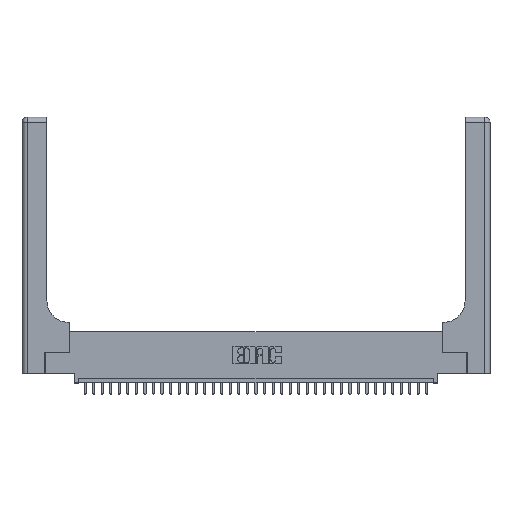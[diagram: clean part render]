
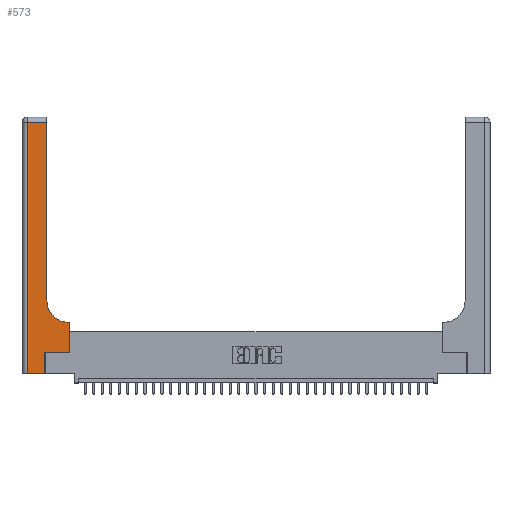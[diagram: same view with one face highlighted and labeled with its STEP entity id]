
A CAD part, top view. The second image highlights one B-rep face of the part: STEP entity #573.
In plain terms, the highlighted planar face has unit normal (0, 0, 1).
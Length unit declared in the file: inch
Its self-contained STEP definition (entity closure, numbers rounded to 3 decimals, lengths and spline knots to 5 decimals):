
#573 = ADVANCED_FACE ( 'NONE', ( #34009 ), #28757, .F. ) ;
#732 = DIRECTION ( 'NONE',  ( 0., 1., 0. ) ) ;
#1636 = VECTOR ( 'NONE', #17524, 39.37008 ) ;
#2463 = CARTESIAN_POINT ( 'NONE',  ( 0.06, 2.94, 0.37 ) ) ;
#3347 = DIRECTION ( 'NONE',  ( 0., -1., 0. ) ) ;
#3861 = CARTESIAN_POINT ( 'NONE',  ( 0.269, 0., 0.37 ) ) ;
#3871 = DIRECTION ( 'NONE',  ( 0., 0., -1. ) ) ;
#4919 = DIRECTION ( 'NONE',  ( 0., 0., -1. ) ) ;
#5036 = CARTESIAN_POINT ( 'NONE',  ( 0.5415, 0.6, 0.37 ) ) ;
#5107 = ORIENTED_EDGE ( 'NONE', *, *, #7528, .T. ) ;
#5230 = EDGE_CURVE ( 'NONE', #20240, #35021, #26653, .T. ) ;
#5284 = CARTESIAN_POINT ( 'NONE',  ( 0.5415, 0.85, 0.37 ) ) ;
#5801 = CARTESIAN_POINT ( 'NONE',  ( 0.269, 0.25, 0.37 ) ) ;
#6693 = CARTESIAN_POINT ( 'NONE',  ( 0.5585, 0.25, 0.37 ) ) ;
#7074 = EDGE_CURVE ( 'NONE', #24769, #20240, #18142, .T. ) ;
#7220 = CARTESIAN_POINT ( 'NONE',  ( 0.2915, 0.85, 0.37 ) ) ;
#7409 = EDGE_LOOP ( 'NONE', ( #34728, #28143, #26007, #19621, #34927, #36185, #23797, #20882, #5107 ) ) ;
#7528 = EDGE_CURVE ( 'NONE', #23286, #25486, #25134, .T. ) ;
#8420 = LINE ( 'NONE', #15697, #35168 ) ;
#8437 = CARTESIAN_POINT ( 'NONE',  ( 0., 0., 0.37 ) ) ;
#8805 = DIRECTION ( 'NONE',  ( -1., 0., 0. ) ) ;
#10621 = DIRECTION ( 'NONE',  ( 1., 0., 0. ) ) ;
#10842 = EDGE_CURVE ( 'NONE', #25486, #23081, #34946, .T. ) ;
#12001 = DIRECTION ( 'NONE',  ( 0., 1., 0. ) ) ;
#14422 = VECTOR ( 'NONE', #12001, 39.37008 ) ;
#14959 = DIRECTION ( 'NONE',  ( -1., 0., 0. ) ) ;
#15079 = CARTESIAN_POINT ( 'NONE',  ( 0., 3., 0.37 ) ) ;
#15422 = EDGE_CURVE ( 'NONE', #32567, #24769, #21526, .T. ) ;
#15676 = DIRECTION ( 'NONE',  ( 1., 0., 0. ) ) ;
#15697 = CARTESIAN_POINT ( 'NONE',  ( 0., 2.94, 0.37 ) ) ;
#16866 = EDGE_CURVE ( 'NONE', #35021, #20359, #33232, .T. ) ;
#17463 = LINE ( 'NONE', #6693, #18391 ) ;
#17524 = DIRECTION ( 'NONE',  ( 1., 0., 0. ) ) ;
#17814 = CARTESIAN_POINT ( 'NONE',  ( 0.2915, 3., 0.37 ) ) ;
#18142 = LINE ( 'NONE', #8437, #30452 ) ;
#18391 = VECTOR ( 'NONE', #26775, 39.37008 ) ;
#19621 = ORIENTED_EDGE ( 'NONE', *, *, #7074, .T. ) ;
#20240 = VERTEX_POINT ( 'NONE', #3861 ) ;
#20359 = VERTEX_POINT ( 'NONE', #24331 ) ;
#20882 = ORIENTED_EDGE ( 'NONE', *, *, #34352, .T. ) ;
#21526 = LINE ( 'NONE', #35166, #31147 ) ;
#21652 = EDGE_CURVE ( 'NONE', #23081, #32567, #8420, .T. ) ;
#22621 = CARTESIAN_POINT ( 'NONE',  ( 0.5585, 0.6, 0.37 ) ) ;
#23081 = VERTEX_POINT ( 'NONE', #34076 ) ;
#23286 = VERTEX_POINT ( 'NONE', #5036 ) ;
#23545 = CARTESIAN_POINT ( 'NONE',  ( 0.269, 0., 0.37 ) ) ;
#23676 = EDGE_CURVE ( 'NONE', #20359, #28381, #17463, .T. ) ;
#23797 = ORIENTED_EDGE ( 'NONE', *, *, #23676, .T. ) ;
#24331 = CARTESIAN_POINT ( 'NONE',  ( 0.5585, 0.25, 0.37 ) ) ;
#24769 = VERTEX_POINT ( 'NONE', #27180 ) ;
#25134 = CIRCLE ( 'NONE', #28511, 0.25 ) ;
#25486 = VERTEX_POINT ( 'NONE', #7220 ) ;
#26007 = ORIENTED_EDGE ( 'NONE', *, *, #15422, .T. ) ;
#26653 = LINE ( 'NONE', #23545, #29741 ) ;
#26775 = DIRECTION ( 'NONE',  ( 0., 1., 0. ) ) ;
#27180 = CARTESIAN_POINT ( 'NONE',  ( 0.06, 0., 0.37 ) ) ;
#28143 = ORIENTED_EDGE ( 'NONE', *, *, #21652, .T. ) ;
#28381 = VERTEX_POINT ( 'NONE', #22621 ) ;
#28511 = AXIS2_PLACEMENT_3D ( 'NONE', #5284, #4919, #10621 ) ;
#28757 = PLANE ( 'NONE',  #32927 ) ;
#29741 = VECTOR ( 'NONE', #732, 39.37008 ) ;
#29873 = DIRECTION ( 'NONE',  ( -1., 0., 0. ) ) ;
#30452 = VECTOR ( 'NONE', #15676, 39.37008 ) ;
#31011 = CARTESIAN_POINT ( 'NONE',  ( 0.2915, 0.6, 0.37 ) ) ;
#31147 = VECTOR ( 'NONE', #3347, 39.37008 ) ;
#32567 = VERTEX_POINT ( 'NONE', #2463 ) ;
#32927 = AXIS2_PLACEMENT_3D ( 'NONE', #15079, #3871, #14959 ) ;
#33232 = LINE ( 'NONE', #34324, #1636 ) ;
#33653 = VECTOR ( 'NONE', #8805, 39.37008 ) ;
#34009 = FACE_OUTER_BOUND ( 'NONE', #7409, .T. ) ;
#34076 = CARTESIAN_POINT ( 'NONE',  ( 0.2915, 2.94, 0.37 ) ) ;
#34324 = CARTESIAN_POINT ( 'NONE',  ( 0.269, 0.25, 0.37 ) ) ;
#34352 = EDGE_CURVE ( 'NONE', #28381, #23286, #34541, .T. ) ;
#34541 = LINE ( 'NONE', #31011, #33653 ) ;
#34728 = ORIENTED_EDGE ( 'NONE', *, *, #10842, .T. ) ;
#34927 = ORIENTED_EDGE ( 'NONE', *, *, #5230, .T. ) ;
#34946 = LINE ( 'NONE', #17814, #14422 ) ;
#35021 = VERTEX_POINT ( 'NONE', #5801 ) ;
#35166 = CARTESIAN_POINT ( 'NONE',  ( 0.06, 3., 0.37 ) ) ;
#35168 = VECTOR ( 'NONE', #29873, 39.37008 ) ;
#36185 = ORIENTED_EDGE ( 'NONE', *, *, #16866, .T. ) ;
